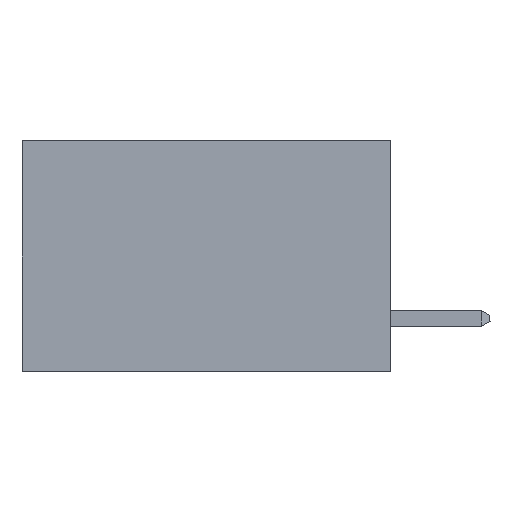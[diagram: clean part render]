
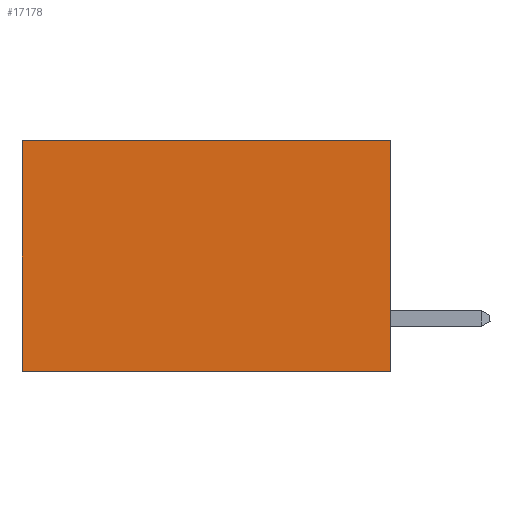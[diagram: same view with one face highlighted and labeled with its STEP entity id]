
A CAD part, left-side view. The second image highlights one B-rep face of the part: STEP entity #17178.
In plain terms, the highlighted planar face has unit normal (-1, 0, 0).
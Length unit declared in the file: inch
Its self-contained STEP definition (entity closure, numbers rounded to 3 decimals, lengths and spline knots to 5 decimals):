
#178 = VECTOR ( 'NONE', #29248, 39.37008 ) ;
#619 = VECTOR ( 'NONE', #21515, 39.37008 ) ;
#930 = EDGE_CURVE ( 'NONE', #24963, #11350, #25793, .T. ) ;
#2076 = EDGE_CURVE ( 'NONE', #24963, #8449, #5082, .T. ) ;
#2168 = CARTESIAN_POINT ( 'NONE',  ( 0.277, 0., -0.37 ) ) ;
#5082 = LINE ( 'NONE', #12374, #23149 ) ;
#6885 = ORIENTED_EDGE ( 'NONE', *, *, #930, .F. ) ;
#7084 = CARTESIAN_POINT ( 'NONE',  ( 0.277, 0.59, 0. ) ) ;
#8152 = CARTESIAN_POINT ( 'NONE',  ( 0.277, 0., -0.37 ) ) ;
#8449 = VERTEX_POINT ( 'NONE', #7084 ) ;
#8793 = VERTEX_POINT ( 'NONE', #25215 ) ;
#9511 = DIRECTION ( 'NONE',  ( 0., 0., -1. ) ) ;
#11350 = VERTEX_POINT ( 'NONE', #8152 ) ;
#11706 = PLANE ( 'NONE',  #16525 ) ;
#12066 = DIRECTION ( 'NONE',  ( 0., 1., 0. ) ) ;
#12374 = CARTESIAN_POINT ( 'NONE',  ( 0.277, 0., 0. ) ) ;
#12802 = LINE ( 'NONE', #24549, #178 ) ;
#14005 = CARTESIAN_POINT ( 'NONE',  ( 0.277, 0., 0. ) ) ;
#15853 = VECTOR ( 'NONE', #28015, 39.37008 ) ;
#16525 = AXIS2_PLACEMENT_3D ( 'NONE', #21228, #23592, #9511 ) ;
#17178 = ADVANCED_FACE ( 'NONE', ( #24456 ), #11706, .F. ) ;
#18242 = EDGE_LOOP ( 'NONE', ( #20248, #28900, #6885, #26239 ) ) ;
#19169 = EDGE_CURVE ( 'NONE', #11350, #8793, #22187, .T. ) ;
#20248 = ORIENTED_EDGE ( 'NONE', *, *, #21872, .T. ) ;
#20761 = CARTESIAN_POINT ( 'NONE',  ( 0.277, 0., -0.37 ) ) ;
#21228 = CARTESIAN_POINT ( 'NONE',  ( 0.277, 0., -0.37 ) ) ;
#21515 = DIRECTION ( 'NONE',  ( 0., 0., -1. ) ) ;
#21872 = EDGE_CURVE ( 'NONE', #8449, #8793, #12802, .T. ) ;
#22187 = LINE ( 'NONE', #2168, #15853 ) ;
#23149 = VECTOR ( 'NONE', #12066, 39.37008 ) ;
#23592 = DIRECTION ( 'NONE',  ( 1., 0., 0. ) ) ;
#24456 = FACE_OUTER_BOUND ( 'NONE', #18242, .T. ) ;
#24549 = CARTESIAN_POINT ( 'NONE',  ( 0.277, 0.59, -0.37 ) ) ;
#24963 = VERTEX_POINT ( 'NONE', #14005 ) ;
#25215 = CARTESIAN_POINT ( 'NONE',  ( 0.277, 0.59, -0.37 ) ) ;
#25793 = LINE ( 'NONE', #20761, #619 ) ;
#26239 = ORIENTED_EDGE ( 'NONE', *, *, #2076, .T. ) ;
#28015 = DIRECTION ( 'NONE',  ( 0., 1., 0. ) ) ;
#28900 = ORIENTED_EDGE ( 'NONE', *, *, #19169, .F. ) ;
#29248 = DIRECTION ( 'NONE',  ( 0., 0., -1. ) ) ;
